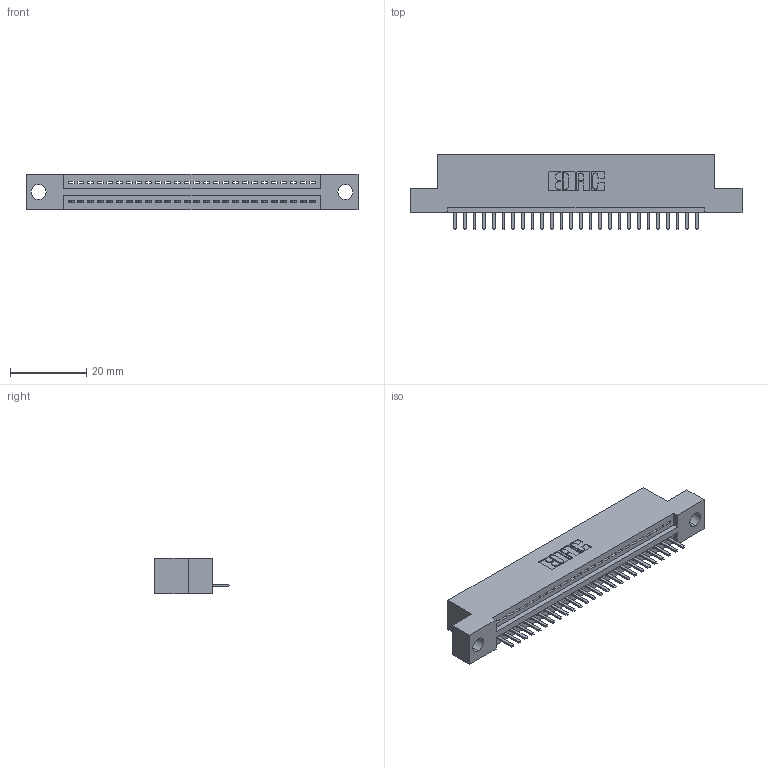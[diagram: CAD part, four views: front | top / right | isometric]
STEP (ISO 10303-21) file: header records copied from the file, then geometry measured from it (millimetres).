
FILE_DESCRIPTION (( 'STEP AP203' ), '1' );
FILE_NAME ('395-026-520-104.STEP', '2021-05-31T14:37:00', ( '' ), ( '' ), 'SwSTEP 2.0', 'SolidWorks 2020', '' );
FILE_SCHEMA (( 'CONFIG_CONTROL_DESIGN' ));
Length unit declared in the file: inch
Products named in the file (3): 395-026-520-104; 345-292-001_345-293-120; 345 Part_Flush Mounting Lugs - 0.156 Dia-TI
Assembly tree (27 placements, depth 2):
  395-026-520-104
    345 Part_Flush Mounting Lugs - 0.156 Dia-TI
    345-292-001_345-293-120  x26
Bounding box: 87.25 x 19.68 x 9.4 mm (x, y, z)
Volume: 7975.2 mm3; surface area: 9978.7 mm2
Topology: 27 solids, 27 shells, 1752 faces, 5161 edges, 3370 vertices
Faces by surface type: plane 1186, cylinder 566
Entity records: 22255 total; most frequent: CARTESIAN_POINT 3876, ORIENTED_EDGE 3822, DIRECTION 3395, EDGE_CURVE 1911, VECTOR 1671, LINE 1671, VERTEX_POINT 1270, AXIS2_PLACEMENT_3D 862
